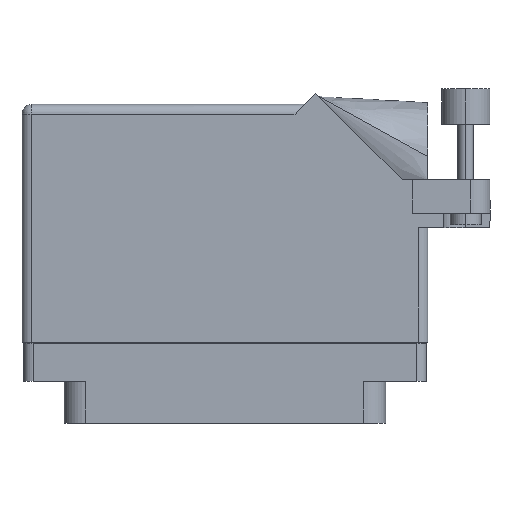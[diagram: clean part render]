
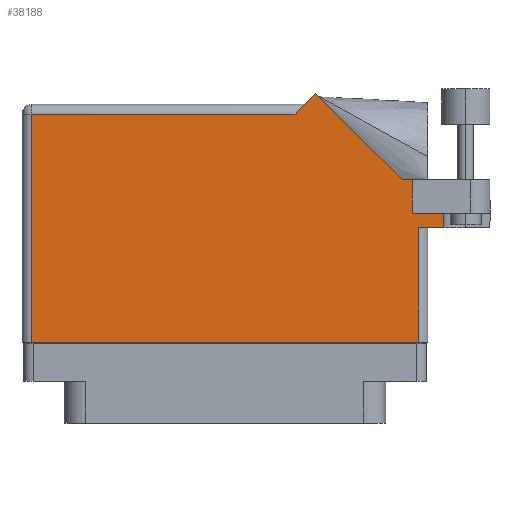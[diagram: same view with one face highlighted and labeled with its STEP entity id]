
A CAD part, front view. The second image highlights one B-rep face of the part: STEP entity #38188.
In plain terms, the highlighted face is planar.
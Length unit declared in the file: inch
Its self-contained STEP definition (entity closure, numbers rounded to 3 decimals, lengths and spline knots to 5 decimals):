
#402 = CARTESIAN_POINT ( 'NONE',  ( 0.58371, 1.50071, 0.455 ) ) ;
#1094 = CARTESIAN_POINT ( 'NONE',  ( 1.306, 0.637, 0.455 ) ) ;
#1396 = CARTESIAN_POINT ( 'NONE',  ( -1.306, -0.1, 0.455 ) ) ;
#2053 = DIRECTION ( 'NONE',  ( 0., 1., 0. ) ) ;
#2424 = DIRECTION ( 'NONE',  ( 0., 1., 0. ) ) ;
#2765 = EDGE_CURVE ( 'NONE', #47506, #3713, #2969, .T. ) ;
#2969 = LINE ( 'NONE', #42891, #24302 ) ;
#3517 = ORIENTED_EDGE ( 'NONE', *, *, #29971, .T. ) ;
#3713 = VERTEX_POINT ( 'NONE', #18948 ) ;
#5150 = DIRECTION ( 'NONE',  ( -0.707, 0.707, 0. ) ) ;
#6600 = CARTESIAN_POINT ( 'NONE',  ( 1.206, 0.731, 0.455 ) ) ;
#7028 = DIRECTION ( 'NONE',  ( 0., -1., 0. ) ) ;
#7417 = ORIENTED_EDGE ( 'NONE', *, *, #7768, .T. ) ;
#7764 = LINE ( 'NONE', #8289, #36581 ) ;
#7768 = EDGE_CURVE ( 'NONE', #22442, #27531, #29613, .T. ) ;
#7810 = LINE ( 'NONE', #43241, #46352 ) ;
#7971 = FACE_OUTER_BOUND ( 'NONE', #25267, .T. ) ;
#8289 = CARTESIAN_POINT ( 'NONE',  ( 1.206, 0.731, 0.455 ) ) ;
#8859 = VECTOR ( 'NONE', #5150, 39.37008 ) ;
#9121 = CARTESIAN_POINT ( 'NONE',  ( 1.14042, 0.944, 0.455 ) ) ;
#10581 = EDGE_CURVE ( 'NONE', #13077, #12512, #17900, .T. ) ;
#12450 = CARTESIAN_POINT ( 'NONE',  ( -1.306, 1.43, 0.455 ) ) ;
#12512 = VERTEX_POINT ( 'NONE', #43727 ) ;
#12662 = ORIENTED_EDGE ( 'NONE', *, *, #10581, .T. ) ;
#12814 = CARTESIAN_POINT ( 'NONE',  ( 0.513, 1.43, 0.455 ) ) ;
#13077 = VERTEX_POINT ( 'NONE', #6600 ) ;
#13871 = CARTESIAN_POINT ( 'NONE',  ( 1.4075, 0.731, 0.455 ) ) ;
#13873 = LINE ( 'NONE', #12814, #27560 ) ;
#15205 = ORIENTED_EDGE ( 'NONE', *, *, #52053, .F. ) ;
#16108 = EDGE_CURVE ( 'NONE', #13077, #49417, #7764, .T. ) ;
#17900 = LINE ( 'NONE', #29541, #19772 ) ;
#17986 = VERTEX_POINT ( 'NONE', #47511 ) ;
#18920 = ORIENTED_EDGE ( 'NONE', *, *, #34677, .T. ) ;
#18935 = CARTESIAN_POINT ( 'NONE',  ( 1.706, 0.944, 0.455 ) ) ;
#18948 = CARTESIAN_POINT ( 'NONE',  ( -1.244, -0.1, 0.455 ) ) ;
#19772 = VECTOR ( 'NONE', #2053, 39.37008 ) ;
#19817 = VERTEX_POINT ( 'NONE', #402 ) ;
#20187 = CARTESIAN_POINT ( 'NONE',  ( -1.306, 1.368, 0.455 ) ) ;
#22442 = VERTEX_POINT ( 'NONE', #40773 ) ;
#22494 = LINE ( 'NONE', #31192, #30337 ) ;
#22918 = EDGE_CURVE ( 'NONE', #3713, #27427, #41824, .T. ) ;
#22994 = ORIENTED_EDGE ( 'NONE', *, *, #23116, .T. ) ;
#23011 = CARTESIAN_POINT ( 'NONE',  ( 1.4075, 0.637, 0.455 ) ) ;
#23116 = EDGE_CURVE ( 'NONE', #27427, #22442, #22494, .T. ) ;
#24302 = VECTOR ( 'NONE', #43676, 39.37008 ) ;
#25267 = EDGE_LOOP ( 'NONE', ( #48038, #22994, #7417, #15205, #30395, #12662, #29617, #3517, #18920, #47858, #28521 ) ) ;
#25334 = EDGE_CURVE ( 'NONE', #12512, #32476, #26083, .T. ) ;
#26083 = LINE ( 'NONE', #18935, #31351 ) ;
#26859 = DIRECTION ( 'NONE',  ( -1., 0., 0. ) ) ;
#27427 = VERTEX_POINT ( 'NONE', #37067 ) ;
#27531 = VERTEX_POINT ( 'NONE', #23011 ) ;
#27560 = VECTOR ( 'NONE', #45082, 39.37008 ) ;
#28521 = ORIENTED_EDGE ( 'NONE', *, *, #2765, .T. ) ;
#28870 = VECTOR ( 'NONE', #36308, 39.37008 ) ;
#29191 = LINE ( 'NONE', #9121, #8859 ) ;
#29541 = CARTESIAN_POINT ( 'NONE',  ( 1.206, 0.731, 0.455 ) ) ;
#29613 = LINE ( 'NONE', #1094, #34051 ) ;
#29617 = ORIENTED_EDGE ( 'NONE', *, *, #25334, .T. ) ;
#29971 = EDGE_CURVE ( 'NONE', #32476, #19817, #29191, .T. ) ;
#30337 = VECTOR ( 'NONE', #2424, 39.37008 ) ;
#30395 = ORIENTED_EDGE ( 'NONE', *, *, #16108, .F. ) ;
#31192 = CARTESIAN_POINT ( 'NONE',  ( 1.244, 0.637, 0.455 ) ) ;
#31351 = VECTOR ( 'NONE', #26859, 39.37008 ) ;
#32118 = AXIS2_PLACEMENT_3D ( 'NONE', #12450, #32517, #48683 ) ;
#32476 = VERTEX_POINT ( 'NONE', #36744 ) ;
#32517 = DIRECTION ( 'NONE',  ( 0., 0., -1. ) ) ;
#33830 = DIRECTION ( 'NONE',  ( 1., 0., 0. ) ) ;
#34051 = VECTOR ( 'NONE', #33830, 39.37008 ) ;
#34677 = EDGE_CURVE ( 'NONE', #19817, #17986, #13873, .T. ) ;
#36233 = VECTOR ( 'NONE', #37848, 39.37008 ) ;
#36308 = DIRECTION ( 'NONE',  ( -1., 0., 0. ) ) ;
#36574 = LINE ( 'NONE', #20187, #28870 ) ;
#36581 = VECTOR ( 'NONE', #40009, 39.37008 ) ;
#36744 = CARTESIAN_POINT ( 'NONE',  ( 1.14042, 0.944, 0.455 ) ) ;
#37067 = CARTESIAN_POINT ( 'NONE',  ( 1.244, -0.1, 0.455 ) ) ;
#37848 = DIRECTION ( 'NONE',  ( 1., 0., 0. ) ) ;
#38188 = ADVANCED_FACE ( 'NONE', ( #7971 ), #48160, .F. ) ;
#40009 = DIRECTION ( 'NONE',  ( 1., 0., 0. ) ) ;
#40614 = CARTESIAN_POINT ( 'NONE',  ( -1.244, 1.368, 0.455 ) ) ;
#40773 = CARTESIAN_POINT ( 'NONE',  ( 1.244, 0.637, 0.455 ) ) ;
#41824 = LINE ( 'NONE', #1396, #36233 ) ;
#41937 = EDGE_CURVE ( 'NONE', #17986, #47506, #36574, .T. ) ;
#42891 = CARTESIAN_POINT ( 'NONE',  ( -1.244, -0.1, 0.455 ) ) ;
#43241 = CARTESIAN_POINT ( 'NONE',  ( 1.4075, 1.06177, 0.455 ) ) ;
#43676 = DIRECTION ( 'NONE',  ( 0., -1., 0. ) ) ;
#43727 = CARTESIAN_POINT ( 'NONE',  ( 1.206, 0.944, 0.455 ) ) ;
#45082 = DIRECTION ( 'NONE',  ( -0.707, -0.707, 0. ) ) ;
#46352 = VECTOR ( 'NONE', #7028, 39.37008 ) ;
#47506 = VERTEX_POINT ( 'NONE', #40614 ) ;
#47511 = CARTESIAN_POINT ( 'NONE',  ( 0.451, 1.368, 0.455 ) ) ;
#47858 = ORIENTED_EDGE ( 'NONE', *, *, #41937, .T. ) ;
#48038 = ORIENTED_EDGE ( 'NONE', *, *, #22918, .T. ) ;
#48160 = PLANE ( 'NONE',  #32118 ) ;
#48683 = DIRECTION ( 'NONE',  ( -1., 0., 0. ) ) ;
#49417 = VERTEX_POINT ( 'NONE', #13871 ) ;
#52053 = EDGE_CURVE ( 'NONE', #49417, #27531, #7810, .T. ) ;
